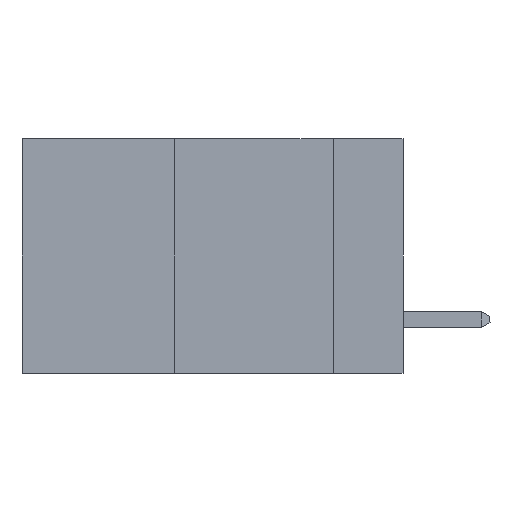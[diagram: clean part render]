
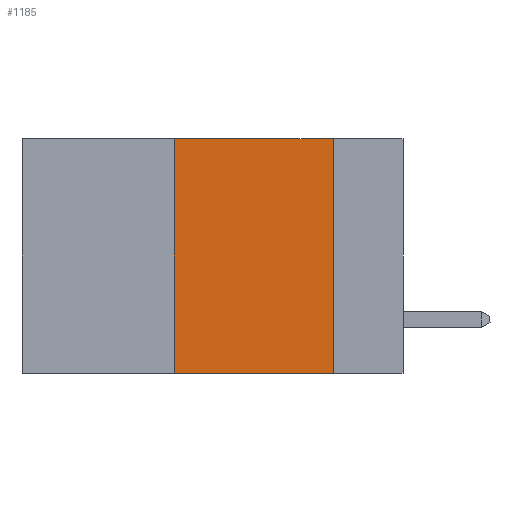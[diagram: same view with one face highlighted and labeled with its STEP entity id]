
A CAD part, left-side view. The second image highlights one B-rep face of the part: STEP entity #1185.
In plain terms, the highlighted planar face has unit normal (-1, 0, 0).
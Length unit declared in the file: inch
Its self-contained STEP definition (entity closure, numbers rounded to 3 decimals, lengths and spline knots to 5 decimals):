
#331 = FACE_OUTER_BOUND ( 'NONE', #15370, .T. ) ;
#899 = ORIENTED_EDGE ( 'NONE', *, *, #2526, .T. ) ;
#1185 = ADVANCED_FACE ( 'NONE', ( #331 ), #3656, .F. ) ;
#1247 = CARTESIAN_POINT ( 'NONE',  ( 0., 0.36, 0. ) ) ;
#1373 = CARTESIAN_POINT ( 'NONE',  ( 0., 0.11, -0.37 ) ) ;
#1590 = EDGE_CURVE ( 'NONE', #14432, #14539, #12412, .T. ) ;
#1971 = AXIS2_PLACEMENT_3D ( 'NONE', #7990, #11027, #13228 ) ;
#2384 = EDGE_CURVE ( 'NONE', #14539, #11494, #12571, .T. ) ;
#2526 = EDGE_CURVE ( 'NONE', #14432, #4849, #2664, .T. ) ;
#2664 = LINE ( 'NONE', #7060, #9339 ) ;
#2744 = CARTESIAN_POINT ( 'NONE',  ( 0., 0.11, 0. ) ) ;
#2922 = DIRECTION ( 'NONE',  ( 0., 0., -1. ) ) ;
#3656 = PLANE ( 'NONE',  #1971 ) ;
#4232 = DIRECTION ( 'NONE',  ( 0., -1., 0. ) ) ;
#4849 = VERTEX_POINT ( 'NONE', #1373 ) ;
#5459 = LINE ( 'NONE', #9507, #8604 ) ;
#6322 = CARTESIAN_POINT ( 'NONE',  ( 0., 0.6, 0. ) ) ;
#6779 = VECTOR ( 'NONE', #12592, 39.37008 ) ;
#7060 = CARTESIAN_POINT ( 'NONE',  ( 0., 0.6, -0.37 ) ) ;
#7990 = CARTESIAN_POINT ( 'NONE',  ( 0., 0.6, 0. ) ) ;
#8604 = VECTOR ( 'NONE', #2922, 39.37008 ) ;
#9072 = EDGE_CURVE ( 'NONE', #11494, #4849, #5459, .T. ) ;
#9339 = VECTOR ( 'NONE', #4232, 39.37008 ) ;
#9507 = CARTESIAN_POINT ( 'NONE',  ( 0., 0.11, 0. ) ) ;
#10683 = CARTESIAN_POINT ( 'NONE',  ( 0., 0.36, -0.37 ) ) ;
#11027 = DIRECTION ( 'NONE',  ( 1., 0., 0. ) ) ;
#11494 = VERTEX_POINT ( 'NONE', #2744 ) ;
#12412 = LINE ( 'NONE', #1247, #6779 ) ;
#12571 = LINE ( 'NONE', #6322, #12934 ) ;
#12592 = DIRECTION ( 'NONE',  ( 0., 0., 1. ) ) ;
#12934 = VECTOR ( 'NONE', #15970, 39.37008 ) ;
#13143 = ORIENTED_EDGE ( 'NONE', *, *, #1590, .F. ) ;
#13228 = DIRECTION ( 'NONE',  ( 0., 0., -1. ) ) ;
#14371 = CARTESIAN_POINT ( 'NONE',  ( 0., 0.36, 0. ) ) ;
#14432 = VERTEX_POINT ( 'NONE', #10683 ) ;
#14539 = VERTEX_POINT ( 'NONE', #14371 ) ;
#14873 = ORIENTED_EDGE ( 'NONE', *, *, #2384, .F. ) ;
#14938 = ORIENTED_EDGE ( 'NONE', *, *, #9072, .F. ) ;
#15370 = EDGE_LOOP ( 'NONE', ( #14938, #14873, #13143, #899 ) ) ;
#15970 = DIRECTION ( 'NONE',  ( 0., -1., 0. ) ) ;
